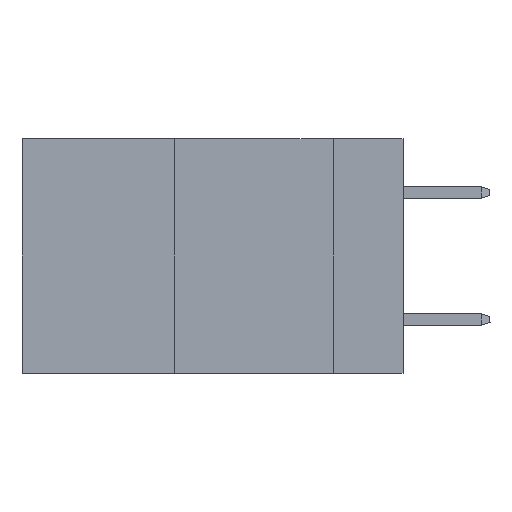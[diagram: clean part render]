
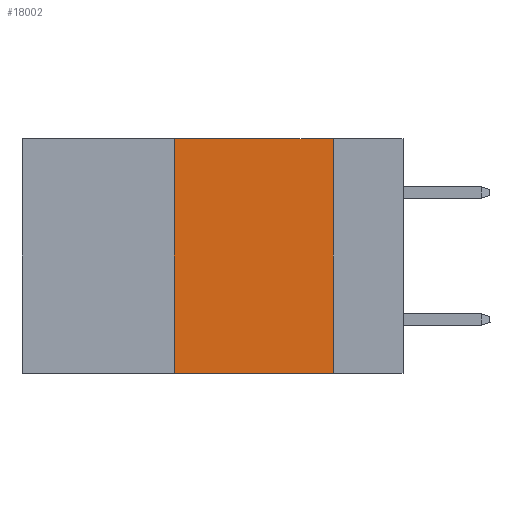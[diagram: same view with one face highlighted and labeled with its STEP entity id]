
A CAD part, left-side view. The second image highlights one B-rep face of the part: STEP entity #18002.
In plain terms, the highlighted planar face has unit normal (-1, 0, 0).
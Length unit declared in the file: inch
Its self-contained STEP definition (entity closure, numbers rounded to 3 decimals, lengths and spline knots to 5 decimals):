
#378 = ORIENTED_EDGE ( 'NONE', *, *, #13111, .F. ) ;
#1151 = CARTESIAN_POINT ( 'NONE',  ( 0., 0.11, -0.37 ) ) ;
#1266 = DIRECTION ( 'NONE',  ( 0., -1., 0. ) ) ;
#3909 = EDGE_CURVE ( 'NONE', #21415, #26476, #22448, .T. ) ;
#4256 = VECTOR ( 'NONE', #9459, 39.37008 ) ;
#6603 = DIRECTION ( 'NONE',  ( 0., 0., 1. ) ) ;
#8302 = DIRECTION ( 'NONE',  ( 0., 0., -1. ) ) ;
#8722 = CARTESIAN_POINT ( 'NONE',  ( 0., 0.36, 0. ) ) ;
#9421 = CARTESIAN_POINT ( 'NONE',  ( 0., 0.36, 0. ) ) ;
#9459 = DIRECTION ( 'NONE',  ( 0., -1., 0. ) ) ;
#11697 = LINE ( 'NONE', #26676, #23006 ) ;
#12501 = ORIENTED_EDGE ( 'NONE', *, *, #3909, .T. ) ;
#13111 = EDGE_CURVE ( 'NONE', #21415, #23046, #26395, .T. ) ;
#13152 = DIRECTION ( 'NONE',  ( 1., 0., 0. ) ) ;
#13174 = EDGE_CURVE ( 'NONE', #23046, #25528, #11697, .T. ) ;
#13576 = FACE_OUTER_BOUND ( 'NONE', #14608, .T. ) ;
#14266 = CARTESIAN_POINT ( 'NONE',  ( 0., 0.6, -0.37 ) ) ;
#14608 = EDGE_LOOP ( 'NONE', ( #17186, #14634, #378, #12501 ) ) ;
#14634 = ORIENTED_EDGE ( 'NONE', *, *, #13174, .F. ) ;
#14673 = EDGE_CURVE ( 'NONE', #25528, #26476, #19053, .T. ) ;
#15258 = CARTESIAN_POINT ( 'NONE',  ( 0., 0.11, 0. ) ) ;
#16798 = CARTESIAN_POINT ( 'NONE',  ( 0., 0.36, -0.37 ) ) ;
#17186 = ORIENTED_EDGE ( 'NONE', *, *, #14673, .F. ) ;
#18002 = ADVANCED_FACE ( 'NONE', ( #13576 ), #26582, .F. ) ;
#19053 = LINE ( 'NONE', #27642, #27162 ) ;
#19097 = AXIS2_PLACEMENT_3D ( 'NONE', #24323, #13152, #22043 ) ;
#21415 = VERTEX_POINT ( 'NONE', #16798 ) ;
#22043 = DIRECTION ( 'NONE',  ( 0., 0., -1. ) ) ;
#22448 = LINE ( 'NONE', #14266, #4256 ) ;
#23006 = VECTOR ( 'NONE', #1266, 39.37008 ) ;
#23046 = VERTEX_POINT ( 'NONE', #9421 ) ;
#23429 = VECTOR ( 'NONE', #6603, 39.37008 ) ;
#24323 = CARTESIAN_POINT ( 'NONE',  ( 0., 0.6, 0. ) ) ;
#25528 = VERTEX_POINT ( 'NONE', #15258 ) ;
#26395 = LINE ( 'NONE', #8722, #23429 ) ;
#26476 = VERTEX_POINT ( 'NONE', #1151 ) ;
#26582 = PLANE ( 'NONE',  #19097 ) ;
#26676 = CARTESIAN_POINT ( 'NONE',  ( 0., 0.6, 0. ) ) ;
#27162 = VECTOR ( 'NONE', #8302, 39.37008 ) ;
#27642 = CARTESIAN_POINT ( 'NONE',  ( 0., 0.11, 0. ) ) ;
